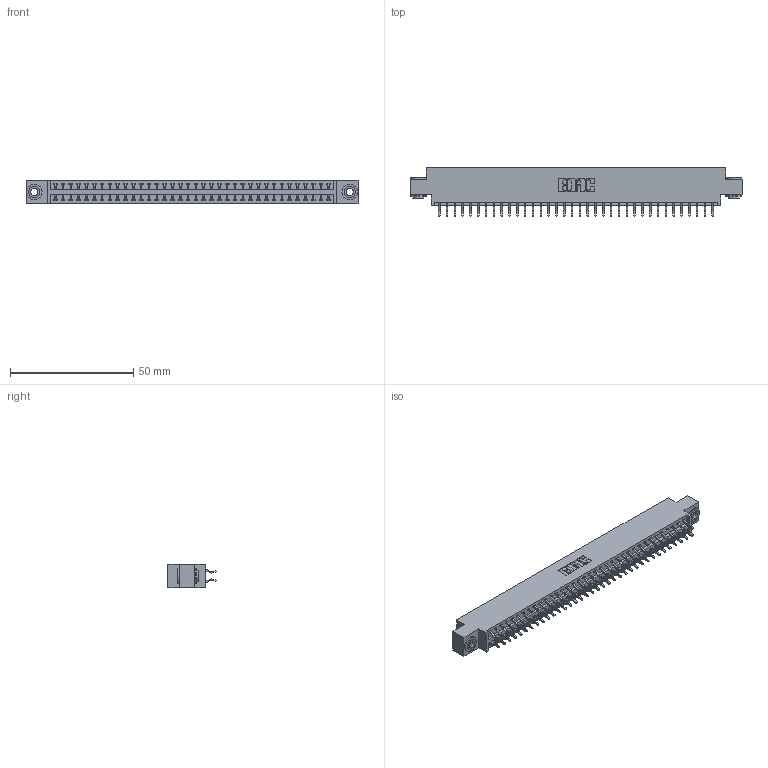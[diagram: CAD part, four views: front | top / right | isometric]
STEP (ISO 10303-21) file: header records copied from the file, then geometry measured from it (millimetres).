
FILE_DESCRIPTION (( 'STEP AP203' ), '1' );
FILE_NAME ('346-072-556-803.STEP', '2018-08-29T01:16:57', ( '' ), ( '' ), 'SwSTEP 2.0', 'SolidWorks 2016', '' );
FILE_SCHEMA (( 'CONFIG_CONTROL_DESIGN' ));
Length unit declared in the file: inch
Products named in the file (4): 346 Part_0.170 Offset - 0.156 Dia-TH; 345-292-001_556 Tail; 345-250-002_345-250-002-102; 346-072-556-803
Assembly tree (75 placements, depth 2):
  346-072-556-803
    346 Part_0.170 Offset - 0.156 Dia-TH
    345-292-001_556 Tail  x72
    345-250-002_345-250-002-102  x2
Bounding box: 134.87 x 19.57 x 9.4 mm (x, y, z)
Volume: 12967.2 mm3; surface area: 18056.9 mm2
Topology: 75 solids, 75 shells, 4340 faces, 12873 edges, 8482 vertices
Faces by surface type: plane 2898, cylinder 1434, cone 8
Entity records: 25304 total; most frequent: CARTESIAN_POINT 4171, ORIENTED_EDGE 4086, DIRECTION 3745, EDGE_CURVE 2043, VECTOR 1735, LINE 1735, VERTEX_POINT 1358, AXIS2_PLACEMENT_3D 1005
